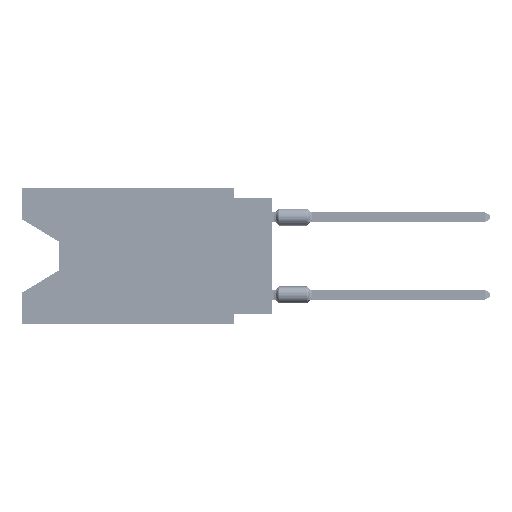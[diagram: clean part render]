
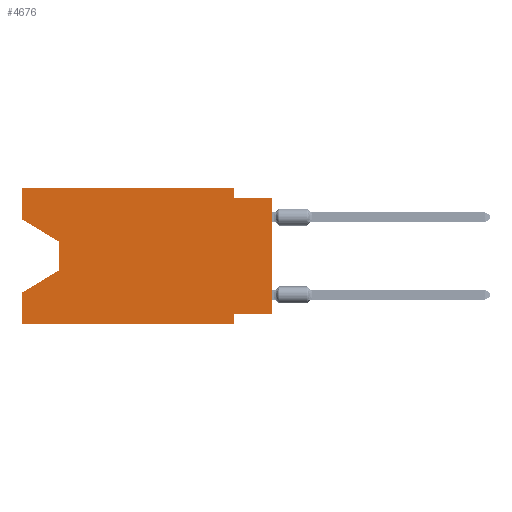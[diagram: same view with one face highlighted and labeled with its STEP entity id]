
A CAD part, left-side view. The second image highlights one B-rep face of the part: STEP entity #4676.
In plain terms, the highlighted planar face has unit normal (-1, 0, 0).
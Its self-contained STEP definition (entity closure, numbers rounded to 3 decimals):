
#195 = DIRECTION ( 'NONE',  ( 0., 0., -1. ) ) ;
#499 = VERTEX_POINT ( 'NONE', #24275 ) ;
#561 = AXIS2_PLACEMENT_3D ( 'NONE', #63805, #11576, #56936 ) ;
#1291 = CARTESIAN_POINT ( 'NONE',  ( 0., 13.97, -5.385 ) ) ;
#1511 = VERTEX_POINT ( 'NONE', #57078 ) ;
#3455 = VECTOR ( 'NONE', #15605, 1000. ) ;
#3844 = VECTOR ( 'NONE', #11382, 1000. ) ;
#3929 = VECTOR ( 'NONE', #15362, 1000. ) ;
#4225 = CARTESIAN_POINT ( 'NONE',  ( 0., 2.54, -0.635 ) ) ;
#4274 = VECTOR ( 'NONE', #195, 1000. ) ;
#4676 = ADVANCED_FACE ( 'NONE', ( #16550 ), #40541, .F. ) ;
#5007 = CARTESIAN_POINT ( 'NONE',  ( 0., 13.97, -5.385 ) ) ;
#5979 = VERTEX_POINT ( 'NONE', #62031 ) ;
#6455 = VERTEX_POINT ( 'NONE', #48823 ) ;
#7718 = EDGE_CURVE ( 'NONE', #27098, #18183, #50299, .T. ) ;
#8523 = ORIENTED_EDGE ( 'NONE', *, *, #63599, .F. ) ;
#8740 = EDGE_CURVE ( 'NONE', #49420, #58364, #48532, .T. ) ;
#9763 = VECTOR ( 'NONE', #75037, 1000. ) ;
#10088 = EDGE_CURVE ( 'NONE', #1511, #27098, #72567, .T. ) ;
#10707 = ORIENTED_EDGE ( 'NONE', *, *, #10088, .F. ) ;
#11382 = DIRECTION ( 'NONE',  ( 0., -1., 0. ) ) ;
#11412 = CARTESIAN_POINT ( 'NONE',  ( 0., 2.54, -8.89 ) ) ;
#11576 = DIRECTION ( 'NONE',  ( 1., 0., 0. ) ) ;
#13120 = DIRECTION ( 'NONE',  ( 0., 0., 1. ) ) ;
#13480 = LINE ( 'NONE', #36722, #38414 ) ;
#13519 = ORIENTED_EDGE ( 'NONE', *, *, #34940, .T. ) ;
#13717 = ORIENTED_EDGE ( 'NONE', *, *, #66776, .T. ) ;
#14916 = EDGE_LOOP ( 'NONE', ( #13717, #69128, #57686, #35527, #13519, #69689, #10707, #62446, #24863, #8523, #44964, #48598 ) ) ;
#15362 = DIRECTION ( 'NONE',  ( 0., 1., 0. ) ) ;
#15605 = DIRECTION ( 'NONE',  ( 0., 0., -1. ) ) ;
#15813 = DIRECTION ( 'NONE',  ( 0., -1., 0. ) ) ;
#16550 = FACE_OUTER_BOUND ( 'NONE', #14916, .T. ) ;
#17376 = EDGE_CURVE ( 'NONE', #6455, #37529, #13480, .T. ) ;
#18183 = VERTEX_POINT ( 'NONE', #11412 ) ;
#18855 = LINE ( 'NONE', #65355, #60040 ) ;
#21068 = LINE ( 'NONE', #43565, #53531 ) ;
#22521 = LINE ( 'NONE', #62921, #42986 ) ;
#22812 = LINE ( 'NONE', #63605, #3844 ) ;
#22924 = DIRECTION ( 'NONE',  ( 0., 0.855, -0.519 ) ) ;
#23788 = CARTESIAN_POINT ( 'NONE',  ( 0., 16.383, -6.852 ) ) ;
#24275 = CARTESIAN_POINT ( 'NONE',  ( 0., 0., -0.635 ) ) ;
#24534 = CARTESIAN_POINT ( 'NONE',  ( 0., 16.383, 0. ) ) ;
#24863 = ORIENTED_EDGE ( 'NONE', *, *, #41157, .F. ) ;
#26131 = CARTESIAN_POINT ( 'NONE',  ( 0., 0., -0.635 ) ) ;
#27098 = VERTEX_POINT ( 'NONE', #41093 ) ;
#29283 = CARTESIAN_POINT ( 'NONE',  ( 0., 16.383, -2.038 ) ) ;
#30015 = VERTEX_POINT ( 'NONE', #46750 ) ;
#34940 = EDGE_CURVE ( 'NONE', #49420, #18183, #21068, .T. ) ;
#35527 = ORIENTED_EDGE ( 'NONE', *, *, #8740, .F. ) ;
#35546 = VECTOR ( 'NONE', #15813, 1000. ) ;
#35596 = DIRECTION ( 'NONE',  ( 0., 0., -1. ) ) ;
#36202 = EDGE_CURVE ( 'NONE', #37529, #58364, #74784, .T. ) ;
#36722 = CARTESIAN_POINT ( 'NONE',  ( 0., 13.97, -3.505 ) ) ;
#37529 = VERTEX_POINT ( 'NONE', #1291 ) ;
#38414 = VECTOR ( 'NONE', #35596, 1000. ) ;
#40541 = PLANE ( 'NONE',  #561 ) ;
#41093 = CARTESIAN_POINT ( 'NONE',  ( 0., 2.54, -8.255 ) ) ;
#41157 = EDGE_CURVE ( 'NONE', #53849, #499, #56587, .T. ) ;
#41337 = VECTOR ( 'NONE', #64568, 1000. ) ;
#42126 = LINE ( 'NONE', #53559, #4274 ) ;
#42986 = VECTOR ( 'NONE', #45385, 1000. ) ;
#43565 = CARTESIAN_POINT ( 'NONE',  ( 0., 16.383, -8.89 ) ) ;
#44964 = ORIENTED_EDGE ( 'NONE', *, *, #68148, .F. ) ;
#45385 = DIRECTION ( 'NONE',  ( 0., 0., 1. ) ) ;
#46425 = LINE ( 'NONE', #29283, #9763 ) ;
#46750 = CARTESIAN_POINT ( 'NONE',  ( 0., 16.383, 0. ) ) ;
#48532 = LINE ( 'NONE', #24534, #41337 ) ;
#48598 = ORIENTED_EDGE ( 'NONE', *, *, #60658, .F. ) ;
#48823 = CARTESIAN_POINT ( 'NONE',  ( 0., 13.97, -3.505 ) ) ;
#49420 = VERTEX_POINT ( 'NONE', #75147 ) ;
#50299 = LINE ( 'NONE', #73558, #3455 ) ;
#52971 = VERTEX_POINT ( 'NONE', #68449 ) ;
#53531 = VECTOR ( 'NONE', #73677, 1000. ) ;
#53559 = CARTESIAN_POINT ( 'NONE',  ( 0., 2.54, 0. ) ) ;
#53849 = VERTEX_POINT ( 'NONE', #4225 ) ;
#54932 = VECTOR ( 'NONE', #22924, 1000. ) ;
#56121 = CARTESIAN_POINT ( 'NONE',  ( 0., 0., -8.255 ) ) ;
#56587 = LINE ( 'NONE', #26131, #35546 ) ;
#56936 = DIRECTION ( 'NONE',  ( 0., 0., -1. ) ) ;
#57078 = CARTESIAN_POINT ( 'NONE',  ( 0., 0., -8.255 ) ) ;
#57686 = ORIENTED_EDGE ( 'NONE', *, *, #36202, .T. ) ;
#58364 = VERTEX_POINT ( 'NONE', #23788 ) ;
#60040 = VECTOR ( 'NONE', #13120, 1000. ) ;
#60658 = EDGE_CURVE ( 'NONE', #52971, #30015, #18855, .T. ) ;
#62031 = CARTESIAN_POINT ( 'NONE',  ( 0., 2.54, 0. ) ) ;
#62446 = ORIENTED_EDGE ( 'NONE', *, *, #71522, .T. ) ;
#62921 = CARTESIAN_POINT ( 'NONE',  ( 0., 0., 0. ) ) ;
#63599 = EDGE_CURVE ( 'NONE', #5979, #53849, #42126, .T. ) ;
#63605 = CARTESIAN_POINT ( 'NONE',  ( 0., 16.383, 0. ) ) ;
#63805 = CARTESIAN_POINT ( 'NONE',  ( 0., 16.383, 0. ) ) ;
#64568 = DIRECTION ( 'NONE',  ( 0., 0., 1. ) ) ;
#65355 = CARTESIAN_POINT ( 'NONE',  ( 0., 16.383, 0. ) ) ;
#66776 = EDGE_CURVE ( 'NONE', #52971, #6455, #46425, .T. ) ;
#68148 = EDGE_CURVE ( 'NONE', #30015, #5979, #22812, .T. ) ;
#68449 = CARTESIAN_POINT ( 'NONE',  ( 0., 16.383, -2.038 ) ) ;
#69128 = ORIENTED_EDGE ( 'NONE', *, *, #17376, .T. ) ;
#69689 = ORIENTED_EDGE ( 'NONE', *, *, #7718, .F. ) ;
#71522 = EDGE_CURVE ( 'NONE', #1511, #499, #22521, .T. ) ;
#72567 = LINE ( 'NONE', #56121, #3929 ) ;
#73558 = CARTESIAN_POINT ( 'NONE',  ( 0., 2.54, -8.89 ) ) ;
#73677 = DIRECTION ( 'NONE',  ( 0., -1., 0. ) ) ;
#74784 = LINE ( 'NONE', #5007, #54932 ) ;
#75037 = DIRECTION ( 'NONE',  ( 0., -0.855, -0.519 ) ) ;
#75147 = CARTESIAN_POINT ( 'NONE',  ( 0., 16.383, -8.89 ) ) ;
